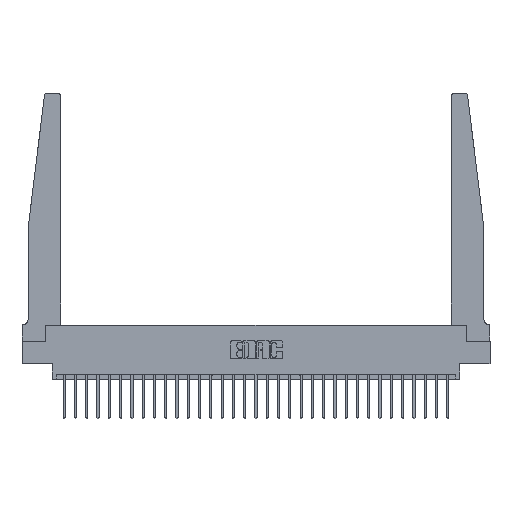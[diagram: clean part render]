
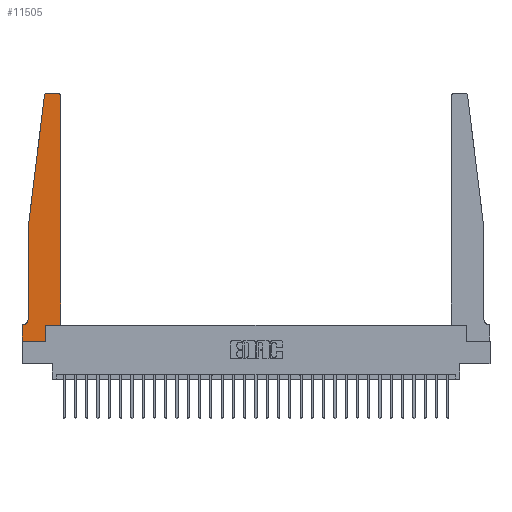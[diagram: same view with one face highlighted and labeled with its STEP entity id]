
A CAD part, top view. The second image highlights one B-rep face of the part: STEP entity #11505.
In plain terms, the highlighted planar face has unit normal (0, 0, 1).
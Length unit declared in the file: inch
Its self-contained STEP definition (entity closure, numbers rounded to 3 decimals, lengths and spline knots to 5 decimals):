
#442 = DIRECTION ( 'NONE',  ( -1., 0., 0. ) ) ;
#490 = ORIENTED_EDGE ( 'NONE', *, *, #6902, .T. ) ;
#1383 = VERTEX_POINT ( 'NONE', #24558 ) ;
#1833 = AXIS2_PLACEMENT_3D ( 'NONE', #18352, #5019, #20583 ) ;
#1865 = CARTESIAN_POINT ( 'NONE',  ( 0.065, 0.2375, 0.37 ) ) ;
#2830 = VECTOR ( 'NONE', #21741, 39.37008 ) ;
#2922 = CARTESIAN_POINT ( 'NONE',  ( 0., 0., 0.37 ) ) ;
#3385 = DIRECTION ( 'NONE',  ( 0., 1., 0. ) ) ;
#3480 = CARTESIAN_POINT ( 'NONE',  ( 0., 0.1875, 0.37 ) ) ;
#3742 = VECTOR ( 'NONE', #11931, 39.37008 ) ;
#3978 = VERTEX_POINT ( 'NONE', #3480 ) ;
#4223 = EDGE_CURVE ( 'NONE', #17112, #3978, #15567, .T. ) ;
#4626 = VECTOR ( 'NONE', #3385, 39.37008 ) ;
#5019 = DIRECTION ( 'NONE',  ( 0., 0., 1. ) ) ;
#5034 = CARTESIAN_POINT ( 'NONE',  ( 0.395, 2.72, 0.37 ) ) ;
#5197 = CARTESIAN_POINT ( 'NONE',  ( 0.425, 2.72, 0.37 ) ) ;
#5204 = CARTESIAN_POINT ( 'NONE',  ( 0.2605, 0.18, 0.37 ) ) ;
#5351 = DIRECTION ( 'NONE',  ( 0., 0., 1. ) ) ;
#5435 = ORIENTED_EDGE ( 'NONE', *, *, #27426, .T. ) ;
#6142 = CARTESIAN_POINT ( 'NONE',  ( 0., 0., 0.37 ) ) ;
#6374 = DIRECTION ( 'NONE',  ( -0.122, -0.992, 0. ) ) ;
#6542 = ORIENTED_EDGE ( 'NONE', *, *, #8727, .T. ) ;
#6546 = VERTEX_POINT ( 'NONE', #19904 ) ;
#6902 = EDGE_CURVE ( 'NONE', #1383, #23337, #17198, .T. ) ;
#7286 = DIRECTION ( 'NONE',  ( 1., 0., 0. ) ) ;
#7402 = ORIENTED_EDGE ( 'NONE', *, *, #24322, .T. ) ;
#7905 = CARTESIAN_POINT ( 'NONE',  ( 0.425, 0.18, 0.37 ) ) ;
#8017 = EDGE_CURVE ( 'NONE', #12259, #17112, #23271, .T. ) ;
#8072 = LINE ( 'NONE', #19705, #13303 ) ;
#8311 = ORIENTED_EDGE ( 'NONE', *, *, #28216, .T. ) ;
#8675 = LINE ( 'NONE', #13547, #19803 ) ;
#8727 = EDGE_CURVE ( 'NONE', #19133, #1383, #12547, .T. ) ;
#8934 = AXIS2_PLACEMENT_3D ( 'NONE', #18671, #5351, #20892 ) ;
#9374 = CARTESIAN_POINT ( 'NONE',  ( 0.25, 2.75, 0.37 ) ) ;
#9503 = CARTESIAN_POINT ( 'NONE',  ( 0.2605, 0.18, 0.37 ) ) ;
#9563 = VERTEX_POINT ( 'NONE', #16312 ) ;
#9696 = LINE ( 'NONE', #2922, #3742 ) ;
#9820 = VECTOR ( 'NONE', #22916, 39.37008 ) ;
#10783 = FACE_OUTER_BOUND ( 'NONE', #23577, .T. ) ;
#11045 = DIRECTION ( 'NONE',  ( 0., 0., -1. ) ) ;
#11074 = ORIENTED_EDGE ( 'NONE', *, *, #8017, .T. ) ;
#11505 = ADVANCED_FACE ( 'NONE', ( #10783 ), #16447, .T. ) ;
#11810 = ORIENTED_EDGE ( 'NONE', *, *, #21394, .T. ) ;
#11857 = CARTESIAN_POINT ( 'NONE',  ( 0., 0., 0.37 ) ) ;
#11931 = DIRECTION ( 'NONE',  ( 0., -1., 0. ) ) ;
#12259 = VERTEX_POINT ( 'NONE', #1865 ) ;
#12547 = LINE ( 'NONE', #21945, #18449 ) ;
#13303 = VECTOR ( 'NONE', #6374, 39.37008 ) ;
#13547 = CARTESIAN_POINT ( 'NONE',  ( 0.065, 1.25, 0.37 ) ) ;
#13558 = CARTESIAN_POINT ( 'NONE',  ( 0.2605, 0., 0.37 ) ) ;
#14332 = EDGE_CURVE ( 'NONE', #9563, #26477, #23734, .T. ) ;
#14581 = ORIENTED_EDGE ( 'NONE', *, *, #19171, .T. ) ;
#14727 = ORIENTED_EDGE ( 'NONE', *, *, #14332, .T. ) ;
#15555 = CARTESIAN_POINT ( 'NONE',  ( 0.015, 0.1875, 0.37 ) ) ;
#15567 = LINE ( 'NONE', #17642, #26578 ) ;
#15589 = VERTEX_POINT ( 'NONE', #22228 ) ;
#15781 = DIRECTION ( 'NONE',  ( 0., -1., 0. ) ) ;
#16312 = CARTESIAN_POINT ( 'NONE',  ( 0.27653, 2.75, 0.37 ) ) ;
#16429 = LINE ( 'NONE', #5204, #9820 ) ;
#16447 = PLANE ( 'NONE',  #8934 ) ;
#17112 = VERTEX_POINT ( 'NONE', #15555 ) ;
#17198 = LINE ( 'NONE', #7905, #4626 ) ;
#17590 = AXIS2_PLACEMENT_3D ( 'NONE', #5034, #20594, #7286 ) ;
#17642 = CARTESIAN_POINT ( 'NONE',  ( 0.065, 0.1875, 0.37 ) ) ;
#17962 = ORIENTED_EDGE ( 'NONE', *, *, #19572, .T. ) ;
#18352 = CARTESIAN_POINT ( 'NONE',  ( 0.27653, 2.72, 0.37 ) ) ;
#18449 = VECTOR ( 'NONE', #24148, 39.37008 ) ;
#18671 = CARTESIAN_POINT ( 'NONE',  ( 0., 0.1875, 0.37 ) ) ;
#19103 = VECTOR ( 'NONE', #442, 39.37008 ) ;
#19133 = VERTEX_POINT ( 'NONE', #9503 ) ;
#19171 = EDGE_CURVE ( 'NONE', #23827, #19133, #16429, .T. ) ;
#19572 = EDGE_CURVE ( 'NONE', #26477, #6546, #8072, .T. ) ;
#19628 = ORIENTED_EDGE ( 'NONE', *, *, #22318, .T. ) ;
#19705 = CARTESIAN_POINT ( 'NONE',  ( 0.065, 1.25, 0.37 ) ) ;
#19803 = VECTOR ( 'NONE', #15781, 39.37008 ) ;
#19825 = LINE ( 'NONE', #9374, #19103 ) ;
#19866 = DIRECTION ( 'NONE',  ( -1., 0., 0. ) ) ;
#19904 = CARTESIAN_POINT ( 'NONE',  ( 0.065, 1.25, 0.37 ) ) ;
#20583 = DIRECTION ( 'NONE',  ( 1., 0., 0. ) ) ;
#20594 = DIRECTION ( 'NONE',  ( 0., 0., 1. ) ) ;
#20892 = DIRECTION ( 'NONE',  ( 1., 0., 0. ) ) ;
#20935 = AXIS2_PLACEMENT_3D ( 'NONE', #24276, #11045, #26503 ) ;
#21394 = EDGE_CURVE ( 'NONE', #6546, #12259, #8675, .T. ) ;
#21741 = DIRECTION ( 'NONE',  ( 1., 0., 0. ) ) ;
#21945 = CARTESIAN_POINT ( 'NONE',  ( 0.425, 0.18, 0.37 ) ) ;
#22228 = CARTESIAN_POINT ( 'NONE',  ( 0.395, 2.75, 0.37 ) ) ;
#22318 = EDGE_CURVE ( 'NONE', #3978, #24658, #9696, .T. ) ;
#22472 = CIRCLE ( 'NONE', #17590, 0.03 ) ;
#22916 = DIRECTION ( 'NONE',  ( 0., 1., 0. ) ) ;
#23271 = CIRCLE ( 'NONE', #20935, 0.05 ) ;
#23337 = VERTEX_POINT ( 'NONE', #5197 ) ;
#23577 = EDGE_LOOP ( 'NONE', ( #5435, #14727, #17962, #11810, #11074, #26800, #19628, #7402, #14581, #6542, #490, #8311 ) ) ;
#23734 = CIRCLE ( 'NONE', #1833, 0.03 ) ;
#23827 = VERTEX_POINT ( 'NONE', #13558 ) ;
#24148 = DIRECTION ( 'NONE',  ( 1., 0., 0. ) ) ;
#24276 = CARTESIAN_POINT ( 'NONE',  ( 0.015, 0.2375, 0.37 ) ) ;
#24322 = EDGE_CURVE ( 'NONE', #24658, #23827, #27123, .T. ) ;
#24558 = CARTESIAN_POINT ( 'NONE',  ( 0.425, 0.18, 0.37 ) ) ;
#24658 = VERTEX_POINT ( 'NONE', #11857 ) ;
#25644 = CARTESIAN_POINT ( 'NONE',  ( 0.24675, 2.72367, 0.37 ) ) ;
#26477 = VERTEX_POINT ( 'NONE', #25644 ) ;
#26503 = DIRECTION ( 'NONE',  ( -1., 0., 0. ) ) ;
#26578 = VECTOR ( 'NONE', #19866, 39.37008 ) ;
#26800 = ORIENTED_EDGE ( 'NONE', *, *, #4223, .T. ) ;
#27123 = LINE ( 'NONE', #6142, #2830 ) ;
#27426 = EDGE_CURVE ( 'NONE', #15589, #9563, #19825, .T. ) ;
#28216 = EDGE_CURVE ( 'NONE', #23337, #15589, #22472, .T. ) ;
